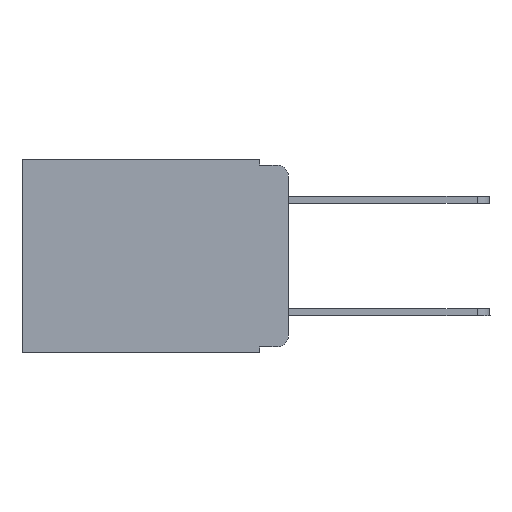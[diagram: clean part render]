
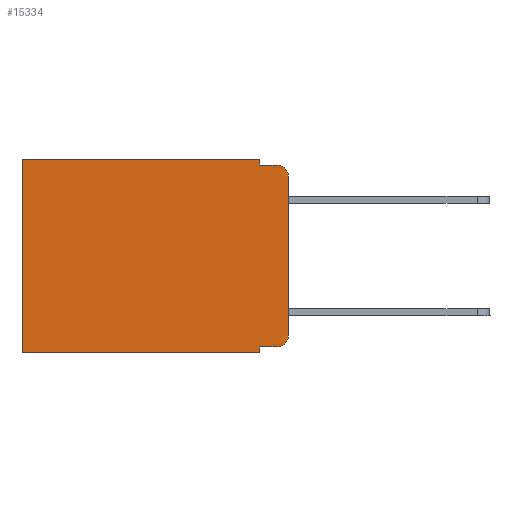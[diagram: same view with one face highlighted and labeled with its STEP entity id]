
A CAD part, left-side view. The second image highlights one B-rep face of the part: STEP entity #15334.
In plain terms, the highlighted planar face has unit normal (-1, 0, 0).
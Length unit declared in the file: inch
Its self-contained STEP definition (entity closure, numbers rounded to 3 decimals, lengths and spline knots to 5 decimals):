
#27 = VERTEX_POINT ( 'NONE', #1452 ) ;
#39 = CARTESIAN_POINT ( 'NONE',  ( 0.298, 0.051, -0.01 ) ) ;
#290 = CARTESIAN_POINT ( 'NONE',  ( 0.298, 0.02, -0.313 ) ) ;
#297 = VERTEX_POINT ( 'NONE', #18168 ) ;
#513 = VERTEX_POINT ( 'NONE', #14115 ) ;
#547 = ORIENTED_EDGE ( 'NONE', *, *, #13452, .T. ) ;
#553 = DIRECTION ( 'NONE',  ( 0., -1., 0. ) ) ;
#1296 = EDGE_CURVE ( 'NONE', #297, #5391, #3560, .T. ) ;
#1422 = DIRECTION ( 'NONE',  ( 0., 0., -1. ) ) ;
#1449 = DIRECTION ( 'NONE',  ( 0., 0., -1. ) ) ;
#1452 = CARTESIAN_POINT ( 'NONE',  ( 0.298, 0., -0.313 ) ) ;
#1523 = CARTESIAN_POINT ( 'NONE',  ( 0.298, 0., 0. ) ) ;
#1552 = DIRECTION ( 'NONE',  ( 0., 0., -1. ) ) ;
#1725 = CARTESIAN_POINT ( 'NONE',  ( 0.298, 0.473, 0. ) ) ;
#1754 = DIRECTION ( 'NONE',  ( 0., -1., 0. ) ) ;
#2165 = CARTESIAN_POINT ( 'NONE',  ( 0.298, 0.051, -0.333 ) ) ;
#2254 = ORIENTED_EDGE ( 'NONE', *, *, #13936, .F. ) ;
#2474 = VECTOR ( 'NONE', #553, 39.37008 ) ;
#2564 = VERTEX_POINT ( 'NONE', #6753 ) ;
#3103 = DIRECTION ( 'NONE',  ( 0., 0., -1. ) ) ;
#3193 = EDGE_LOOP ( 'NONE', ( #2254, #12759, #16461, #20452, #9240, #14344, #18599, #18694, #6834, #547 ) ) ;
#3283 = CARTESIAN_POINT ( 'NONE',  ( 0.298, 0.051, -0.343 ) ) ;
#3560 = LINE ( 'NONE', #39, #7703 ) ;
#3562 = CARTESIAN_POINT ( 'NONE',  ( 0.298, 0.473, 0. ) ) ;
#3585 = EDGE_CURVE ( 'NONE', #13751, #4844, #18305, .T. ) ;
#3790 = LINE ( 'NONE', #13454, #8739 ) ;
#3812 = CARTESIAN_POINT ( 'NONE',  ( 0.298, 0., -0.343 ) ) ;
#4246 = EDGE_CURVE ( 'NONE', #13751, #4432, #8764, .T. ) ;
#4432 = VERTEX_POINT ( 'NONE', #3283 ) ;
#4844 = VERTEX_POINT ( 'NONE', #18402 ) ;
#5074 = EDGE_CURVE ( 'NONE', #513, #5391, #14159, .T. ) ;
#5380 = DIRECTION ( 'NONE',  ( 0., 0., -1. ) ) ;
#5391 = VERTEX_POINT ( 'NONE', #11099 ) ;
#5404 = LINE ( 'NONE', #3812, #11127 ) ;
#5706 = DIRECTION ( 'NONE',  ( 0., 0., -1. ) ) ;
#5995 = EDGE_CURVE ( 'NONE', #10408, #20079, #11647, .T. ) ;
#6753 = CARTESIAN_POINT ( 'NONE',  ( 0.298, 0.051, 0. ) ) ;
#6754 = DIRECTION ( 'NONE',  ( -1., 0., 0. ) ) ;
#6834 = ORIENTED_EDGE ( 'NONE', *, *, #3585, .T. ) ;
#7354 = CIRCLE ( 'NONE', #12467, 0.02 ) ;
#7703 = VECTOR ( 'NONE', #1754, 39.37008 ) ;
#7927 = LINE ( 'NONE', #16084, #12497 ) ;
#7990 = DIRECTION ( 'NONE',  ( 1., 0., 0. ) ) ;
#8044 = AXIS2_PLACEMENT_3D ( 'NONE', #16020, #17840, #3103 ) ;
#8739 = VECTOR ( 'NONE', #5380, 39.37008 ) ;
#8764 = LINE ( 'NONE', #20112, #19522 ) ;
#9240 = ORIENTED_EDGE ( 'NONE', *, *, #17585, .T. ) ;
#10408 = VERTEX_POINT ( 'NONE', #1725 ) ;
#11099 = CARTESIAN_POINT ( 'NONE',  ( 0.298, 0.02, -0.01 ) ) ;
#11127 = VECTOR ( 'NONE', #13787, 39.37008 ) ;
#11251 = DIRECTION ( 'NONE',  ( 0., 1., 0. ) ) ;
#11390 = PLANE ( 'NONE',  #19955 ) ;
#11647 = LINE ( 'NONE', #3562, #19701 ) ;
#12467 = AXIS2_PLACEMENT_3D ( 'NONE', #290, #6754, #13271 ) ;
#12497 = VECTOR ( 'NONE', #1552, 39.37008 ) ;
#12759 = ORIENTED_EDGE ( 'NONE', *, *, #5074, .T. ) ;
#12842 = CARTESIAN_POINT ( 'NONE',  ( 0.298, 0., 0. ) ) ;
#13271 = DIRECTION ( 'NONE',  ( 0., 0., -1. ) ) ;
#13452 = EDGE_CURVE ( 'NONE', #4844, #27, #7354, .T. ) ;
#13454 = CARTESIAN_POINT ( 'NONE',  ( 0.298, 0.051, 0. ) ) ;
#13640 = EDGE_CURVE ( 'NONE', #4432, #20079, #5404, .T. ) ;
#13751 = VERTEX_POINT ( 'NONE', #17598 ) ;
#13787 = DIRECTION ( 'NONE',  ( 0., 1., 0. ) ) ;
#13936 = EDGE_CURVE ( 'NONE', #513, #27, #7927, .T. ) ;
#14043 = EDGE_CURVE ( 'NONE', #2564, #297, #3790, .T. ) ;
#14115 = CARTESIAN_POINT ( 'NONE',  ( 0.298, 0., -0.03 ) ) ;
#14159 = CIRCLE ( 'NONE', #8044, 0.02 ) ;
#14344 = ORIENTED_EDGE ( 'NONE', *, *, #5995, .T. ) ;
#14375 = FACE_OUTER_BOUND ( 'NONE', #3193, .T. ) ;
#14727 = CARTESIAN_POINT ( 'NONE',  ( 0.298, 0.473, -0.343 ) ) ;
#15334 = ADVANCED_FACE ( 'NONE', ( #14375 ), #11390, .F. ) ;
#15893 = LINE ( 'NONE', #12842, #20301 ) ;
#16020 = CARTESIAN_POINT ( 'NONE',  ( 0.298, 0.02, -0.03 ) ) ;
#16084 = CARTESIAN_POINT ( 'NONE',  ( 0.298, 0., 0. ) ) ;
#16461 = ORIENTED_EDGE ( 'NONE', *, *, #1296, .F. ) ;
#17585 = EDGE_CURVE ( 'NONE', #2564, #10408, #15893, .T. ) ;
#17598 = CARTESIAN_POINT ( 'NONE',  ( 0.298, 0.051, -0.333 ) ) ;
#17840 = DIRECTION ( 'NONE',  ( -1., 0., 0. ) ) ;
#18168 = CARTESIAN_POINT ( 'NONE',  ( 0.298, 0.051, -0.01 ) ) ;
#18305 = LINE ( 'NONE', #2165, #2474 ) ;
#18402 = CARTESIAN_POINT ( 'NONE',  ( 0.298, 0.02, -0.333 ) ) ;
#18599 = ORIENTED_EDGE ( 'NONE', *, *, #13640, .F. ) ;
#18694 = ORIENTED_EDGE ( 'NONE', *, *, #4246, .F. ) ;
#19522 = VECTOR ( 'NONE', #5706, 39.37008 ) ;
#19701 = VECTOR ( 'NONE', #1449, 39.37008 ) ;
#19955 = AXIS2_PLACEMENT_3D ( 'NONE', #1523, #7990, #1422 ) ;
#20079 = VERTEX_POINT ( 'NONE', #14727 ) ;
#20112 = CARTESIAN_POINT ( 'NONE',  ( 0.298, 0.051, 0. ) ) ;
#20301 = VECTOR ( 'NONE', #11251, 39.37008 ) ;
#20452 = ORIENTED_EDGE ( 'NONE', *, *, #14043, .F. ) ;
